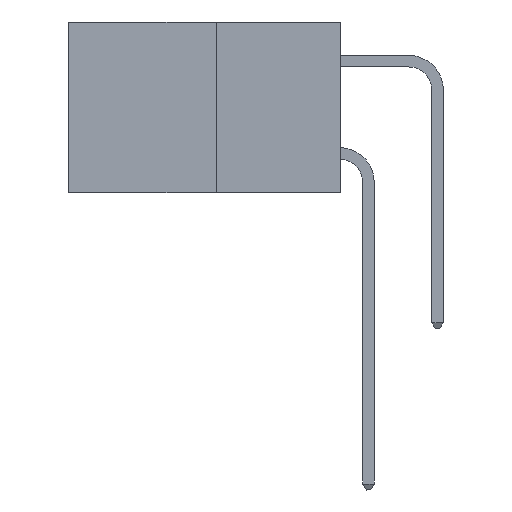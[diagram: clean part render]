
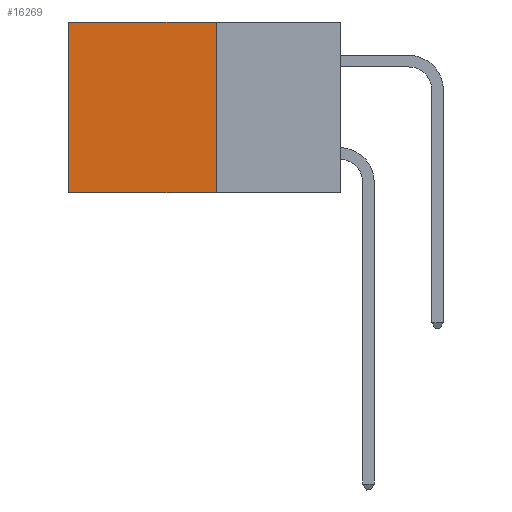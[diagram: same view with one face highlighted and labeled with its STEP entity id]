
A CAD part, left-side view. The second image highlights one B-rep face of the part: STEP entity #16269.
In plain terms, the highlighted planar face has unit normal (-1, 0, 0).
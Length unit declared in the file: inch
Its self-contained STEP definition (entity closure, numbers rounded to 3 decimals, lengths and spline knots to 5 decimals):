
#369 = VERTEX_POINT ( 'NONE', #13918 ) ;
#455 = DIRECTION ( 'NONE',  ( 0., 0., -1. ) ) ;
#1074 = DIRECTION ( 'NONE',  ( 0., 0., -1. ) ) ;
#1741 = EDGE_CURVE ( 'NONE', #14129, #369, #9609, .T. ) ;
#1773 = CARTESIAN_POINT ( 'NONE',  ( 0.277, 0.59, 0. ) ) ;
#2112 = VECTOR ( 'NONE', #2675, 39.37008 ) ;
#2675 = DIRECTION ( 'NONE',  ( 0., 0., -1. ) ) ;
#3322 = ORIENTED_EDGE ( 'NONE', *, *, #13160, .T. ) ;
#3834 = PLANE ( 'NONE',  #15515 ) ;
#3909 = VECTOR ( 'NONE', #14684, 39.37008 ) ;
#4299 = EDGE_LOOP ( 'NONE', ( #3322, #12941, #7793, #15103 ) ) ;
#4494 = VERTEX_POINT ( 'NONE', #10697 ) ;
#6179 = LINE ( 'NONE', #17106, #9459 ) ;
#6220 = EDGE_CURVE ( 'NONE', #14129, #14446, #16144, .T. ) ;
#7793 = ORIENTED_EDGE ( 'NONE', *, *, #1741, .F. ) ;
#8894 = VECTOR ( 'NONE', #11134, 39.37008 ) ;
#9459 = VECTOR ( 'NONE', #455, 39.37008 ) ;
#9490 = CARTESIAN_POINT ( 'NONE',  ( 0.277, 0.27, 0. ) ) ;
#9531 = DIRECTION ( 'NONE',  ( 1., 0., 0. ) ) ;
#9609 = LINE ( 'NONE', #16789, #2112 ) ;
#10697 = CARTESIAN_POINT ( 'NONE',  ( 0.277, 0.59, -0.37 ) ) ;
#11134 = DIRECTION ( 'NONE',  ( 0., 1., 0. ) ) ;
#11150 = CARTESIAN_POINT ( 'NONE',  ( 0.277, 0.27, 0. ) ) ;
#11924 = CARTESIAN_POINT ( 'NONE',  ( 0.277, 0.27, -0.37 ) ) ;
#12941 = ORIENTED_EDGE ( 'NONE', *, *, #13265, .F. ) ;
#13160 = EDGE_CURVE ( 'NONE', #14446, #4494, #6179, .T. ) ;
#13265 = EDGE_CURVE ( 'NONE', #369, #4494, #15036, .T. ) ;
#13597 = CARTESIAN_POINT ( 'NONE',  ( 0.277, 0.27, -0.37 ) ) ;
#13918 = CARTESIAN_POINT ( 'NONE',  ( 0.277, 0.27, -0.37 ) ) ;
#14129 = VERTEX_POINT ( 'NONE', #9490 ) ;
#14446 = VERTEX_POINT ( 'NONE', #1773 ) ;
#14684 = DIRECTION ( 'NONE',  ( 0., 1., 0. ) ) ;
#15036 = LINE ( 'NONE', #11924, #3909 ) ;
#15103 = ORIENTED_EDGE ( 'NONE', *, *, #6220, .T. ) ;
#15515 = AXIS2_PLACEMENT_3D ( 'NONE', #13597, #9531, #1074 ) ;
#16144 = LINE ( 'NONE', #11150, #8894 ) ;
#16269 = ADVANCED_FACE ( 'NONE', ( #17737 ), #3834, .F. ) ;
#16789 = CARTESIAN_POINT ( 'NONE',  ( 0.277, 0.27, -0.37 ) ) ;
#17106 = CARTESIAN_POINT ( 'NONE',  ( 0.277, 0.59, -0.37 ) ) ;
#17737 = FACE_OUTER_BOUND ( 'NONE', #4299, .T. ) ;
